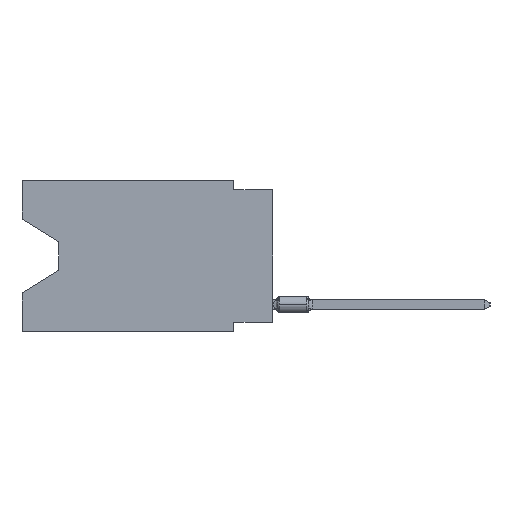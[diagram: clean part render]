
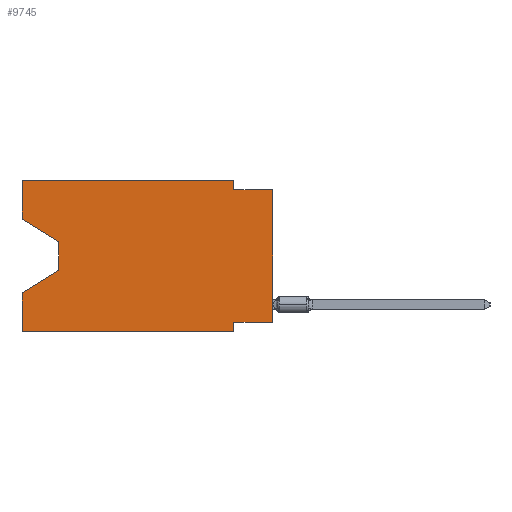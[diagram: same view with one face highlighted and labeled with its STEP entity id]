
A CAD part, left-side view. The second image highlights one B-rep face of the part: STEP entity #9745.
In plain terms, the highlighted planar face has unit normal (-1, 0, 0).
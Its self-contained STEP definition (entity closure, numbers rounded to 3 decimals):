
#74 = CARTESIAN_POINT ( 'NONE',  ( 0., 2.54, 0. ) ) ;
#306 = VECTOR ( 'NONE', #1650, 1000. ) ;
#488 = ORIENTED_EDGE ( 'NONE', *, *, #19918, .T. ) ;
#1338 = DIRECTION ( 'NONE',  ( 1., 0., 0. ) ) ;
#1352 = CARTESIAN_POINT ( 'NONE',  ( 0., 13.97, -4.013 ) ) ;
#1617 = EDGE_CURVE ( 'NONE', #8214, #21602, #8785, .T. ) ;
#1641 = AXIS2_PLACEMENT_3D ( 'NONE', #26530, #1338, #16672 ) ;
#1650 = DIRECTION ( 'NONE',  ( 0., -1., 0. ) ) ;
#1901 = VERTEX_POINT ( 'NONE', #17807 ) ;
#1977 = CARTESIAN_POINT ( 'NONE',  ( 0., 16.383, -9.906 ) ) ;
#2256 = EDGE_LOOP ( 'NONE', ( #13547, #9420, #488, #17600, #6352, #30687, #10368, #11251, #29619, #18699, #18716, #25416 ) ) ;
#2615 = CARTESIAN_POINT ( 'NONE',  ( 0., 0., -9.271 ) ) ;
#2824 = CARTESIAN_POINT ( 'NONE',  ( 0., 0., -0.635 ) ) ;
#3539 = CARTESIAN_POINT ( 'NONE',  ( 0., 2.54, 0. ) ) ;
#4143 = DIRECTION ( 'NONE',  ( 0., -1., 0. ) ) ;
#4314 = LINE ( 'NONE', #26165, #26055 ) ;
#5110 = VECTOR ( 'NONE', #30508, 1000. ) ;
#5168 = DIRECTION ( 'NONE',  ( 0., 0., 1. ) ) ;
#6108 = CARTESIAN_POINT ( 'NONE',  ( 0., 2.54, -0.635 ) ) ;
#6172 = VECTOR ( 'NONE', #11416, 1000. ) ;
#6345 = VERTEX_POINT ( 'NONE', #6948 ) ;
#6352 = ORIENTED_EDGE ( 'NONE', *, *, #1617, .T. ) ;
#6650 = EDGE_CURVE ( 'NONE', #6345, #21602, #26147, .T. ) ;
#6792 = VERTEX_POINT ( 'NONE', #31906 ) ;
#6948 = CARTESIAN_POINT ( 'NONE',  ( 0., 2.54, -9.271 ) ) ;
#7043 = CARTESIAN_POINT ( 'NONE',  ( 0., 0., -9.271 ) ) ;
#7151 = CARTESIAN_POINT ( 'NONE',  ( 0., 13.97, -5.893 ) ) ;
#7530 = DIRECTION ( 'NONE',  ( 0., -1., 0. ) ) ;
#8157 = VERTEX_POINT ( 'NONE', #25186 ) ;
#8214 = VERTEX_POINT ( 'NONE', #26310 ) ;
#8279 = EDGE_CURVE ( 'NONE', #17899, #10004, #8534, .T. ) ;
#8534 = LINE ( 'NONE', #26144, #11881 ) ;
#8785 = LINE ( 'NONE', #1977, #306 ) ;
#9396 = PLANE ( 'NONE',  #1641 ) ;
#9420 = ORIENTED_EDGE ( 'NONE', *, *, #21108, .T. ) ;
#9541 = FACE_OUTER_BOUND ( 'NONE', #2256, .T. ) ;
#9745 = ADVANCED_FACE ( 'NONE', ( #9541 ), #9396, .F. ) ;
#10004 = VERTEX_POINT ( 'NONE', #3539 ) ;
#10368 = ORIENTED_EDGE ( 'NONE', *, *, #23287, .F. ) ;
#10616 = EDGE_CURVE ( 'NONE', #8214, #6792, #22000, .T. ) ;
#10672 = EDGE_CURVE ( 'NONE', #13953, #17899, #24753, .T. ) ;
#10681 = VECTOR ( 'NONE', #7530, 1000. ) ;
#10907 = CARTESIAN_POINT ( 'NONE',  ( 0., 16.383, 0. ) ) ;
#11207 = DIRECTION ( 'NONE',  ( 0., 0., -1. ) ) ;
#11251 = ORIENTED_EDGE ( 'NONE', *, *, #13818, .T. ) ;
#11416 = DIRECTION ( 'NONE',  ( 0., 0., -1. ) ) ;
#11881 = VECTOR ( 'NONE', #4143, 1000. ) ;
#12140 = LINE ( 'NONE', #7151, #31217 ) ;
#12236 = CARTESIAN_POINT ( 'NONE',  ( 0., 16.383, -2.546 ) ) ;
#12281 = CARTESIAN_POINT ( 'NONE',  ( 0., 16.383, 0. ) ) ;
#13061 = VERTEX_POINT ( 'NONE', #2615 ) ;
#13547 = ORIENTED_EDGE ( 'NONE', *, *, #31898, .T. ) ;
#13818 = EDGE_CURVE ( 'NONE', #13061, #21962, #4314, .T. ) ;
#13953 = VERTEX_POINT ( 'NONE', #12236 ) ;
#14474 = LINE ( 'NONE', #7043, #25185 ) ;
#15448 = EDGE_CURVE ( 'NONE', #10004, #26047, #27248, .T. ) ;
#16672 = DIRECTION ( 'NONE',  ( 0., 0., -1. ) ) ;
#16985 = DIRECTION ( 'NONE',  ( 0., 0., 1. ) ) ;
#17094 = DIRECTION ( 'NONE',  ( 0., 0., -1. ) ) ;
#17600 = ORIENTED_EDGE ( 'NONE', *, *, #10616, .F. ) ;
#17807 = CARTESIAN_POINT ( 'NONE',  ( 0., 13.97, -4.013 ) ) ;
#17899 = VERTEX_POINT ( 'NONE', #10907 ) ;
#18698 = CARTESIAN_POINT ( 'NONE',  ( 0., 16.383, -2.546 ) ) ;
#18699 = ORIENTED_EDGE ( 'NONE', *, *, #15448, .F. ) ;
#18716 = ORIENTED_EDGE ( 'NONE', *, *, #8279, .F. ) ;
#19343 = CARTESIAN_POINT ( 'NONE',  ( 0., 0., -0.635 ) ) ;
#19597 = DIRECTION ( 'NONE',  ( 0., 0.855, -0.519 ) ) ;
#19918 = EDGE_CURVE ( 'NONE', #8157, #6792, #12140, .T. ) ;
#20665 = LINE ( 'NONE', #18698, #5110 ) ;
#21012 = DIRECTION ( 'NONE',  ( 0., 0., 1. ) ) ;
#21108 = EDGE_CURVE ( 'NONE', #1901, #8157, #28362, .T. ) ;
#21602 = VERTEX_POINT ( 'NONE', #31865 ) ;
#21962 = VERTEX_POINT ( 'NONE', #19343 ) ;
#22000 = LINE ( 'NONE', #24906, #26015 ) ;
#23287 = EDGE_CURVE ( 'NONE', #13061, #6345, #14474, .T. ) ;
#24753 = LINE ( 'NONE', #12281, #30115 ) ;
#24906 = CARTESIAN_POINT ( 'NONE',  ( 0., 16.383, 0. ) ) ;
#25098 = VECTOR ( 'NONE', #17094, 1000. ) ;
#25185 = VECTOR ( 'NONE', #29014, 1000. ) ;
#25186 = CARTESIAN_POINT ( 'NONE',  ( 0., 13.97, -5.893 ) ) ;
#25416 = ORIENTED_EDGE ( 'NONE', *, *, #10672, .F. ) ;
#25580 = VECTOR ( 'NONE', #11207, 1000. ) ;
#26015 = VECTOR ( 'NONE', #16985, 1000. ) ;
#26047 = VERTEX_POINT ( 'NONE', #6108 ) ;
#26055 = VECTOR ( 'NONE', #21012, 1000. ) ;
#26144 = CARTESIAN_POINT ( 'NONE',  ( 0., 16.383, 0. ) ) ;
#26147 = LINE ( 'NONE', #30831, #6172 ) ;
#26165 = CARTESIAN_POINT ( 'NONE',  ( 0., 0., 0. ) ) ;
#26310 = CARTESIAN_POINT ( 'NONE',  ( 0., 16.383, -9.906 ) ) ;
#26530 = CARTESIAN_POINT ( 'NONE',  ( 0., 16.383, 0. ) ) ;
#26929 = LINE ( 'NONE', #2824, #10681 ) ;
#27248 = LINE ( 'NONE', #74, #25098 ) ;
#27442 = EDGE_CURVE ( 'NONE', #26047, #21962, #26929, .T. ) ;
#28362 = LINE ( 'NONE', #1352, #25580 ) ;
#29014 = DIRECTION ( 'NONE',  ( 0., 1., 0. ) ) ;
#29619 = ORIENTED_EDGE ( 'NONE', *, *, #27442, .F. ) ;
#30115 = VECTOR ( 'NONE', #5168, 1000. ) ;
#30508 = DIRECTION ( 'NONE',  ( 0., -0.855, -0.519 ) ) ;
#30687 = ORIENTED_EDGE ( 'NONE', *, *, #6650, .F. ) ;
#30831 = CARTESIAN_POINT ( 'NONE',  ( 0., 2.54, -9.906 ) ) ;
#31217 = VECTOR ( 'NONE', #19597, 1000. ) ;
#31865 = CARTESIAN_POINT ( 'NONE',  ( 0., 2.54, -9.906 ) ) ;
#31898 = EDGE_CURVE ( 'NONE', #13953, #1901, #20665, .T. ) ;
#31906 = CARTESIAN_POINT ( 'NONE',  ( 0., 16.383, -7.36 ) ) ;
